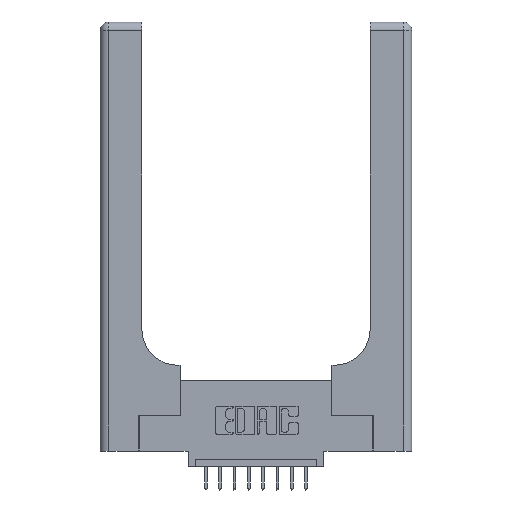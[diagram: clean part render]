
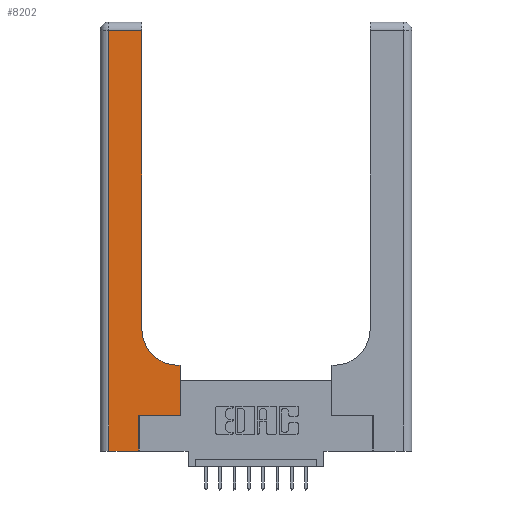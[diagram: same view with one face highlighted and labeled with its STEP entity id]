
A CAD part, top view. The second image highlights one B-rep face of the part: STEP entity #8202.
In plain terms, the highlighted planar face has unit normal (0, 0, 1).
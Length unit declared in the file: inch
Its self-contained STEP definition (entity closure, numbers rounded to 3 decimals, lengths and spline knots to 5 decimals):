
#154 = VECTOR ( 'NONE', #15144, 39.37008 ) ;
#412 = EDGE_CURVE ( 'NONE', #8407, #6787, #3590, .T. ) ;
#499 = DIRECTION ( 'NONE',  ( 0., 1., 0. ) ) ;
#571 = LINE ( 'NONE', #3951, #11990 ) ;
#650 = CARTESIAN_POINT ( 'NONE',  ( 0.2915, 3., 0.37 ) ) ;
#1057 = CARTESIAN_POINT ( 'NONE',  ( 0.5585, 0.6, 0.37 ) ) ;
#1476 = VECTOR ( 'NONE', #7650, 39.37008 ) ;
#1580 = ORIENTED_EDGE ( 'NONE', *, *, #9725, .T. ) ;
#1595 = DIRECTION ( 'NONE',  ( 0., -1., 0. ) ) ;
#1714 = EDGE_CURVE ( 'NONE', #6787, #5883, #2659, .T. ) ;
#2154 = ORIENTED_EDGE ( 'NONE', *, *, #14700, .T. ) ;
#2205 = DIRECTION ( 'NONE',  ( 0., 1., 0. ) ) ;
#2379 = VECTOR ( 'NONE', #499, 39.37008 ) ;
#2659 = LINE ( 'NONE', #7267, #154 ) ;
#2804 = CARTESIAN_POINT ( 'NONE',  ( 0.2915, 0.85, 0.37 ) ) ;
#3074 = VERTEX_POINT ( 'NONE', #3754 ) ;
#3108 = CIRCLE ( 'NONE', #8247, 0.25 ) ;
#3137 = DIRECTION ( 'NONE',  ( 0., 1., 0. ) ) ;
#3590 = LINE ( 'NONE', #6808, #11954 ) ;
#3693 = VECTOR ( 'NONE', #1595, 39.37008 ) ;
#3754 = CARTESIAN_POINT ( 'NONE',  ( 0.269, 0., 0.37 ) ) ;
#3849 = LINE ( 'NONE', #8836, #5983 ) ;
#3873 = CARTESIAN_POINT ( 'NONE',  ( 0.5585, 0.25, 0.37 ) ) ;
#3951 = CARTESIAN_POINT ( 'NONE',  ( 0.269, 0.25, 0.37 ) ) ;
#4309 = DIRECTION ( 'NONE',  ( -1., 0., 0. ) ) ;
#4433 = CARTESIAN_POINT ( 'NONE',  ( 0.269, 0., 0.37 ) ) ;
#4536 = LINE ( 'NONE', #12571, #1476 ) ;
#4913 = ORIENTED_EDGE ( 'NONE', *, *, #9915, .T. ) ;
#5292 = FACE_OUTER_BOUND ( 'NONE', #13701, .T. ) ;
#5396 = DIRECTION ( 'NONE',  ( 0., 0., -1. ) ) ;
#5631 = CARTESIAN_POINT ( 'NONE',  ( 0.06, 0., 0.37 ) ) ;
#5883 = VERTEX_POINT ( 'NONE', #8651 ) ;
#5942 = CARTESIAN_POINT ( 'NONE',  ( 0.5415, 0.85, 0.37 ) ) ;
#5983 = VECTOR ( 'NONE', #14858, 39.37008 ) ;
#5986 = DIRECTION ( 'NONE',  ( 1., 0., 0. ) ) ;
#6263 = ORIENTED_EDGE ( 'NONE', *, *, #412, .T. ) ;
#6394 = CARTESIAN_POINT ( 'NONE',  ( 0.269, 0.25, 0.37 ) ) ;
#6787 = VERTEX_POINT ( 'NONE', #1057 ) ;
#6808 = CARTESIAN_POINT ( 'NONE',  ( 0.5585, 0.25, 0.37 ) ) ;
#7116 = EDGE_CURVE ( 'NONE', #15127, #8407, #571, .T. ) ;
#7267 = CARTESIAN_POINT ( 'NONE',  ( 0.2915, 0.6, 0.37 ) ) ;
#7650 = DIRECTION ( 'NONE',  ( 1., 0., 0. ) ) ;
#7673 = CARTESIAN_POINT ( 'NONE',  ( 0.06, 2.94, 0.37 ) ) ;
#7807 = LINE ( 'NONE', #10314, #3693 ) ;
#7960 = CARTESIAN_POINT ( 'NONE',  ( 0., 3., 0.37 ) ) ;
#8202 = ADVANCED_FACE ( 'NONE', ( #5292 ), #15302, .F. ) ;
#8247 = AXIS2_PLACEMENT_3D ( 'NONE', #5942, #9643, #5986 ) ;
#8407 = VERTEX_POINT ( 'NONE', #3873 ) ;
#8651 = CARTESIAN_POINT ( 'NONE',  ( 0.5415, 0.6, 0.37 ) ) ;
#8836 = CARTESIAN_POINT ( 'NONE',  ( 0., 2.94, 0.37 ) ) ;
#8874 = AXIS2_PLACEMENT_3D ( 'NONE', #7960, #5396, #4309 ) ;
#9179 = ORIENTED_EDGE ( 'NONE', *, *, #1714, .T. ) ;
#9192 = VERTEX_POINT ( 'NONE', #2804 ) ;
#9643 = DIRECTION ( 'NONE',  ( 0., 0., -1. ) ) ;
#9725 = EDGE_CURVE ( 'NONE', #5883, #9192, #3108, .T. ) ;
#9915 = EDGE_CURVE ( 'NONE', #11913, #10653, #3849, .T. ) ;
#10043 = ORIENTED_EDGE ( 'NONE', *, *, #10551, .T. ) ;
#10314 = CARTESIAN_POINT ( 'NONE',  ( 0.06, 3., 0.37 ) ) ;
#10541 = LINE ( 'NONE', #650, #2379 ) ;
#10551 = EDGE_CURVE ( 'NONE', #3074, #15127, #14123, .T. ) ;
#10653 = VERTEX_POINT ( 'NONE', #7673 ) ;
#10740 = ORIENTED_EDGE ( 'NONE', *, *, #15683, .T. ) ;
#11117 = VERTEX_POINT ( 'NONE', #5631 ) ;
#11234 = VECTOR ( 'NONE', #3137, 39.37008 ) ;
#11913 = VERTEX_POINT ( 'NONE', #12433 ) ;
#11954 = VECTOR ( 'NONE', #2205, 39.37008 ) ;
#11990 = VECTOR ( 'NONE', #12860, 39.37008 ) ;
#12433 = CARTESIAN_POINT ( 'NONE',  ( 0.2915, 2.94, 0.37 ) ) ;
#12571 = CARTESIAN_POINT ( 'NONE',  ( 0., 0., 0.37 ) ) ;
#12860 = DIRECTION ( 'NONE',  ( 1., 0., 0. ) ) ;
#13701 = EDGE_LOOP ( 'NONE', ( #14023, #4913, #2154, #10740, #10043, #13907, #6263, #9179, #1580 ) ) ;
#13844 = EDGE_CURVE ( 'NONE', #9192, #11913, #10541, .T. ) ;
#13907 = ORIENTED_EDGE ( 'NONE', *, *, #7116, .T. ) ;
#14023 = ORIENTED_EDGE ( 'NONE', *, *, #13844, .T. ) ;
#14123 = LINE ( 'NONE', #4433, #11234 ) ;
#14700 = EDGE_CURVE ( 'NONE', #10653, #11117, #7807, .T. ) ;
#14858 = DIRECTION ( 'NONE',  ( -1., 0., 0. ) ) ;
#15127 = VERTEX_POINT ( 'NONE', #6394 ) ;
#15144 = DIRECTION ( 'NONE',  ( -1., 0., 0. ) ) ;
#15302 = PLANE ( 'NONE',  #8874 ) ;
#15683 = EDGE_CURVE ( 'NONE', #11117, #3074, #4536, .T. ) ;
